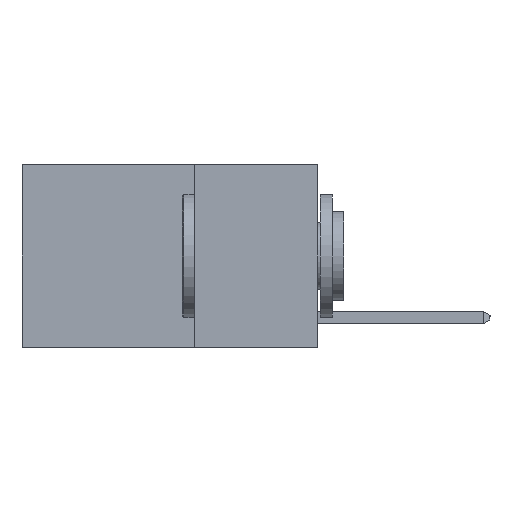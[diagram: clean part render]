
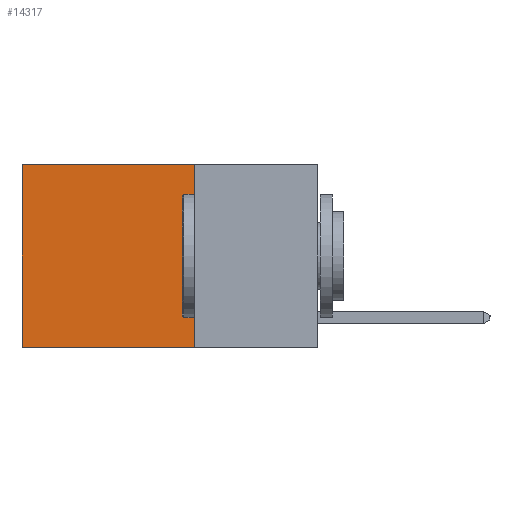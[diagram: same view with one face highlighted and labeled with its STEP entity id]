
A CAD part, left-side view. The second image highlights one B-rep face of the part: STEP entity #14317.
In plain terms, the highlighted planar face has unit normal (-1, 0, 0).
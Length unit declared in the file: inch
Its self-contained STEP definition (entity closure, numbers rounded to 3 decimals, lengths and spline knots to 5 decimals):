
#671 = DIRECTION ( 'NONE',  ( 0., 1., 0. ) ) ;
#876 = VERTEX_POINT ( 'NONE', #10722 ) ;
#1050 = CARTESIAN_POINT ( 'NONE',  ( 0.2625, 0.25, 0. ) ) ;
#1135 = VECTOR ( 'NONE', #6966, 39.37008 ) ;
#1154 = CARTESIAN_POINT ( 'NONE',  ( 0.2625, 0.6, -0.37 ) ) ;
#2169 = CARTESIAN_POINT ( 'NONE',  ( 0.2625, 0.25, 0. ) ) ;
#2499 = VERTEX_POINT ( 'NONE', #8913 ) ;
#2877 = ORIENTED_EDGE ( 'NONE', *, *, #12699, .T. ) ;
#3469 = DIRECTION ( 'NONE',  ( 0., 0., -1. ) ) ;
#3972 = VECTOR ( 'NONE', #3469, 39.37008 ) ;
#4959 = DIRECTION ( 'NONE',  ( 1., 0., 0. ) ) ;
#5262 = ORIENTED_EDGE ( 'NONE', *, *, #9890, .T. ) ;
#5493 = LINE ( 'NONE', #13298, #8510 ) ;
#5822 = CARTESIAN_POINT ( 'NONE',  ( 0.2625, 0.25, 0. ) ) ;
#5884 = ORIENTED_EDGE ( 'NONE', *, *, #14639, .F. ) ;
#6706 = VERTEX_POINT ( 'NONE', #1154 ) ;
#6966 = DIRECTION ( 'NONE',  ( 0., 0., -1. ) ) ;
#7183 = CARTESIAN_POINT ( 'NONE',  ( 0.2625, 0.25, 0. ) ) ;
#8260 = CARTESIAN_POINT ( 'NONE',  ( 0.2625, 0.6, 0. ) ) ;
#8338 = LINE ( 'NONE', #8260, #1135 ) ;
#8491 = DIRECTION ( 'NONE',  ( 0., 1., 0. ) ) ;
#8510 = VECTOR ( 'NONE', #671, 39.37008 ) ;
#8769 = PLANE ( 'NONE',  #15156 ) ;
#8913 = CARTESIAN_POINT ( 'NONE',  ( 0.2625, 0.6, 0. ) ) ;
#9402 = ORIENTED_EDGE ( 'NONE', *, *, #12578, .F. ) ;
#9405 = VECTOR ( 'NONE', #8491, 39.37008 ) ;
#9890 = EDGE_CURVE ( 'NONE', #10501, #2499, #13132, .T. ) ;
#10501 = VERTEX_POINT ( 'NONE', #5822 ) ;
#10722 = CARTESIAN_POINT ( 'NONE',  ( 0.2625, 0.25, -0.37 ) ) ;
#12578 = EDGE_CURVE ( 'NONE', #10501, #876, #14111, .T. ) ;
#12699 = EDGE_CURVE ( 'NONE', #2499, #6706, #8338, .T. ) ;
#13132 = LINE ( 'NONE', #7183, #9405 ) ;
#13298 = CARTESIAN_POINT ( 'NONE',  ( 0.2625, 0.25, -0.37 ) ) ;
#13447 = FACE_OUTER_BOUND ( 'NONE', #16395, .T. ) ;
#13854 = DIRECTION ( 'NONE',  ( 0., 0., -1. ) ) ;
#14111 = LINE ( 'NONE', #2169, #3972 ) ;
#14317 = ADVANCED_FACE ( 'NONE', ( #13447 ), #8769, .F. ) ;
#14639 = EDGE_CURVE ( 'NONE', #876, #6706, #5493, .T. ) ;
#15156 = AXIS2_PLACEMENT_3D ( 'NONE', #1050, #4959, #13854 ) ;
#16395 = EDGE_LOOP ( 'NONE', ( #2877, #5884, #9402, #5262 ) ) ;
